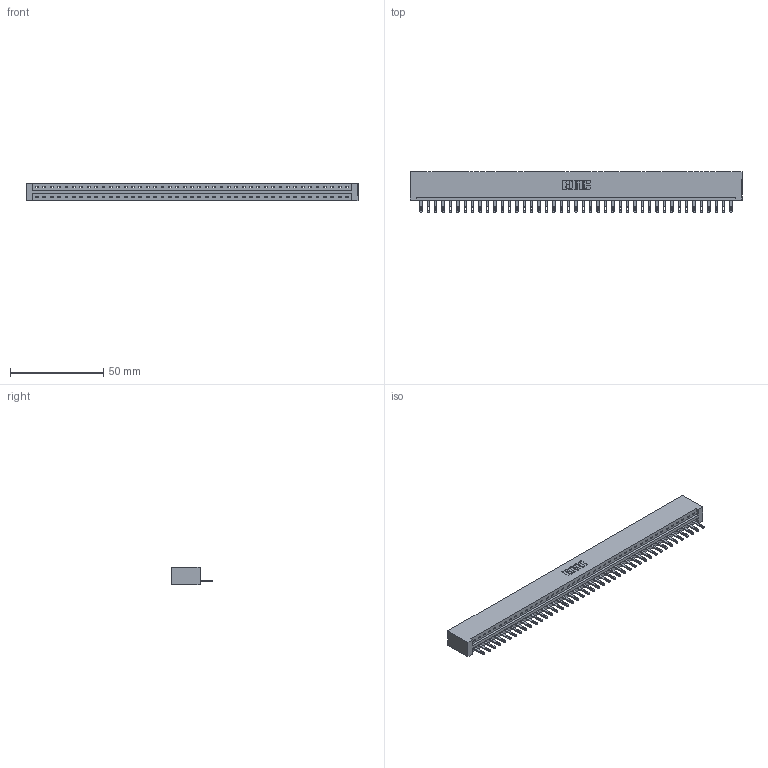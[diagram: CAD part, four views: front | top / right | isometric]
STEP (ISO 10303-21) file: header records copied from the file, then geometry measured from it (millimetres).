
FILE_DESCRIPTION (( 'STEP AP203' ), '1' );
FILE_NAME ('337-043-500-101.STEP', '2019-10-01T22:48:24', ( '' ), ( '' ), 'SwSTEP 2.0', 'SolidWorks 2016', '' );
FILE_SCHEMA (( 'CONFIG_CONTROL_DESIGN' ));
Length unit declared in the file: inch
Products named in the file (3): 337-043-500-101; 345-292-001_345-293-100; 337 Part_No Mounting Lugs
Assembly tree (44 placements, depth 2):
  337-043-500-101
    337 Part_No Mounting Lugs
    345-292-001_345-293-100  x43
Bounding box: 178.26 x 21.85 x 9.4 mm (x, y, z)
Volume: 19304.7 mm3; surface area: 20035.9 mm2
Topology: 44 solids, 44 shells, 2600 faces, 8027 edges, 5350 vertices
Faces by surface type: plane 1786, cylinder 814
Entity records: 31487 total; most frequent: CARTESIAN_POINT 5491, ORIENTED_EDGE 5470, DIRECTION 4613, EDGE_CURVE 2735, LINE 2611, VECTOR 2611, VERTEX_POINT 1822, AXIS2_PLACEMENT_3D 1001
